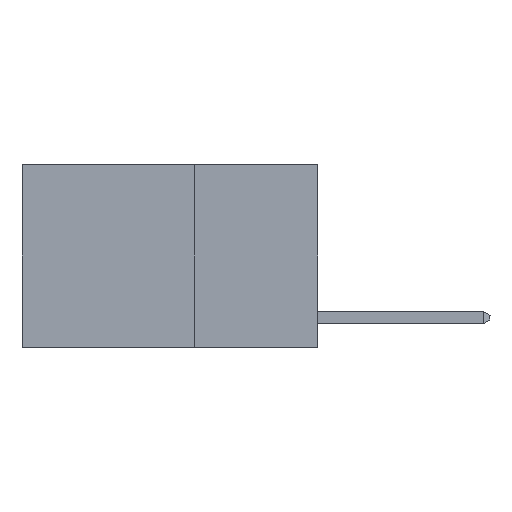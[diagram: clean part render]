
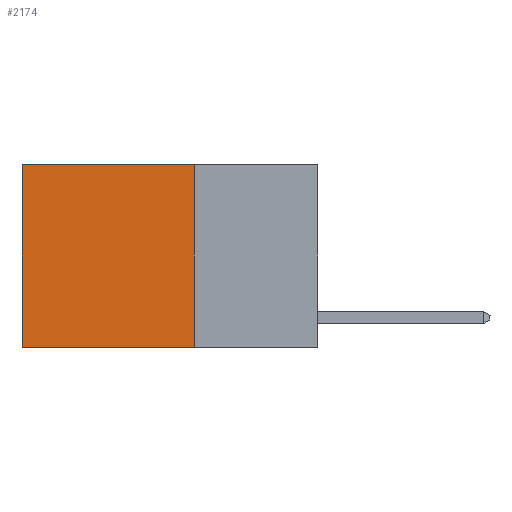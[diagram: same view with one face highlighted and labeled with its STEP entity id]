
A CAD part, left-side view. The second image highlights one B-rep face of the part: STEP entity #2174.
In plain terms, the highlighted planar face has unit normal (-1, 0, 0).
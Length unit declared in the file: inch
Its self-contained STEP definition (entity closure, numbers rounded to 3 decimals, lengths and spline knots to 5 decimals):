
#61 = LINE ( 'NONE', #3806, #3321 ) ;
#760 = ORIENTED_EDGE ( 'NONE', *, *, #9043, .T. ) ;
#1077 = VERTEX_POINT ( 'NONE', #4049 ) ;
#1343 = AXIS2_PLACEMENT_3D ( 'NONE', #11732, #4949, #12843 ) ;
#1792 = VECTOR ( 'NONE', #5503, 39.37008 ) ;
#2174 = ADVANCED_FACE ( 'NONE', ( #2531 ), #9501, .F. ) ;
#2184 = CARTESIAN_POINT ( 'NONE',  ( 0.2625, 0.25, -0.37 ) ) ;
#2198 = VECTOR ( 'NONE', #14824, 39.37008 ) ;
#2531 = FACE_OUTER_BOUND ( 'NONE', #13992, .T. ) ;
#2571 = DIRECTION ( 'NONE',  ( 0., 1., 0. ) ) ;
#3321 = VECTOR ( 'NONE', #11746, 39.37008 ) ;
#3502 = CARTESIAN_POINT ( 'NONE',  ( 0.2625, 0.6, 0. ) ) ;
#3806 = CARTESIAN_POINT ( 'NONE',  ( 0.2625, 0.25, -0.37 ) ) ;
#3996 = VERTEX_POINT ( 'NONE', #11337 ) ;
#4049 = CARTESIAN_POINT ( 'NONE',  ( 0.2625, 0.25, 0. ) ) ;
#4908 = LINE ( 'NONE', #10602, #13198 ) ;
#4949 = DIRECTION ( 'NONE',  ( 1., 0., 0. ) ) ;
#5324 = LINE ( 'NONE', #3502, #2198 ) ;
#5503 = DIRECTION ( 'NONE',  ( 0., 0., -1. ) ) ;
#5868 = EDGE_CURVE ( 'NONE', #1077, #14256, #13615, .T. ) ;
#6037 = VERTEX_POINT ( 'NONE', #11421 ) ;
#6208 = EDGE_CURVE ( 'NONE', #14256, #6037, #61, .T. ) ;
#7739 = ORIENTED_EDGE ( 'NONE', *, *, #11593, .T. ) ;
#9043 = EDGE_CURVE ( 'NONE', #3996, #6037, #5324, .T. ) ;
#9381 = ORIENTED_EDGE ( 'NONE', *, *, #5868, .F. ) ;
#9501 = PLANE ( 'NONE',  #1343 ) ;
#10602 = CARTESIAN_POINT ( 'NONE',  ( 0.2625, 0.25, 0. ) ) ;
#11162 = CARTESIAN_POINT ( 'NONE',  ( 0.2625, 0.25, 0. ) ) ;
#11337 = CARTESIAN_POINT ( 'NONE',  ( 0.2625, 0.6, 0. ) ) ;
#11421 = CARTESIAN_POINT ( 'NONE',  ( 0.2625, 0.6, -0.37 ) ) ;
#11593 = EDGE_CURVE ( 'NONE', #1077, #3996, #4908, .T. ) ;
#11732 = CARTESIAN_POINT ( 'NONE',  ( 0.2625, 0.25, 0. ) ) ;
#11746 = DIRECTION ( 'NONE',  ( 0., 1., 0. ) ) ;
#12222 = ORIENTED_EDGE ( 'NONE', *, *, #6208, .F. ) ;
#12843 = DIRECTION ( 'NONE',  ( 0., 0., -1. ) ) ;
#13198 = VECTOR ( 'NONE', #2571, 39.37008 ) ;
#13615 = LINE ( 'NONE', #11162, #1792 ) ;
#13992 = EDGE_LOOP ( 'NONE', ( #760, #12222, #9381, #7739 ) ) ;
#14256 = VERTEX_POINT ( 'NONE', #2184 ) ;
#14824 = DIRECTION ( 'NONE',  ( 0., 0., -1. ) ) ;
